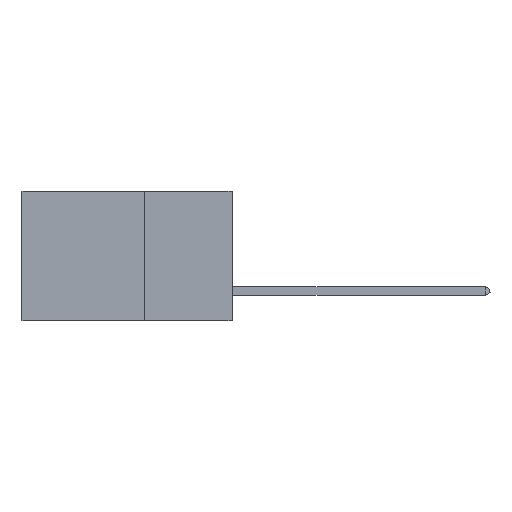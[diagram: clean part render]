
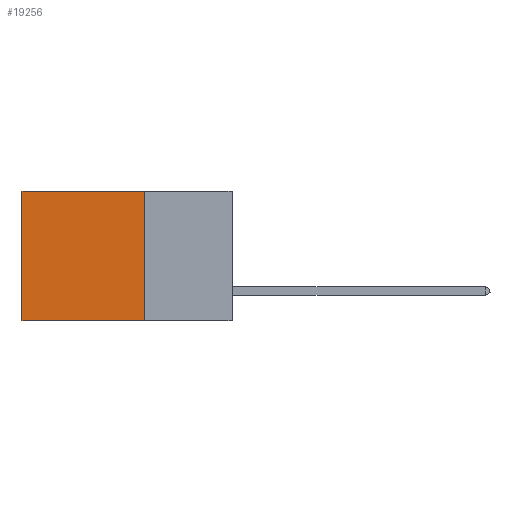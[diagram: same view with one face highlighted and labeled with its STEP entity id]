
A CAD part, left-side view. The second image highlights one B-rep face of the part: STEP entity #19256.
In plain terms, the highlighted planar face has unit normal (-1, 0, 0).
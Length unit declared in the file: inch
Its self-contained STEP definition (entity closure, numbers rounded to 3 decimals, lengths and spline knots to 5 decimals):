
#1192 = EDGE_LOOP ( 'NONE', ( #1279, #43005, #9288, #31970 ) ) ;
#1279 = ORIENTED_EDGE ( 'NONE', *, *, #7587, .T. ) ;
#2018 = CARTESIAN_POINT ( 'NONE',  ( 0.2875, 0.25, 0. ) ) ;
#5462 = AXIS2_PLACEMENT_3D ( 'NONE', #16844, #16388, #23739 ) ;
#7587 = EDGE_CURVE ( 'NONE', #22575, #18100, #30866, .T. ) ;
#8755 = DIRECTION ( 'NONE',  ( 0., 1., 0. ) ) ;
#9239 = DIRECTION ( 'NONE',  ( 0., 0., -1. ) ) ;
#9288 = ORIENTED_EDGE ( 'NONE', *, *, #26504, .F. ) ;
#16388 = DIRECTION ( 'NONE',  ( 1., 0., 0. ) ) ;
#16671 = LINE ( 'NONE', #2018, #36842 ) ;
#16844 = CARTESIAN_POINT ( 'NONE',  ( 0.2875, 0.25, 0. ) ) ;
#18100 = VERTEX_POINT ( 'NONE', #31803 ) ;
#18764 = VECTOR ( 'NONE', #8755, 39.37008 ) ;
#19256 = ADVANCED_FACE ( 'NONE', ( #23884 ), #38470, .F. ) ;
#19267 = DIRECTION ( 'NONE',  ( 0., 0., -1. ) ) ;
#22202 = DIRECTION ( 'NONE',  ( 0., 1., 0. ) ) ;
#22575 = VERTEX_POINT ( 'NONE', #42373 ) ;
#23262 = CARTESIAN_POINT ( 'NONE',  ( 0.2875, 0.25, -0.37 ) ) ;
#23739 = DIRECTION ( 'NONE',  ( 0., 0., -1. ) ) ;
#23884 = FACE_OUTER_BOUND ( 'NONE', #1192, .T. ) ;
#24040 = EDGE_CURVE ( 'NONE', #28176, #22575, #35311, .T. ) ;
#26504 = EDGE_CURVE ( 'NONE', #28176, #43264, #16671, .T. ) ;
#28176 = VERTEX_POINT ( 'NONE', #44977 ) ;
#29634 = CARTESIAN_POINT ( 'NONE',  ( 0.2875, 0.25, 0. ) ) ;
#30866 = LINE ( 'NONE', #41692, #43025 ) ;
#31803 = CARTESIAN_POINT ( 'NONE',  ( 0.2875, 0.6, -0.37 ) ) ;
#31970 = ORIENTED_EDGE ( 'NONE', *, *, #24040, .T. ) ;
#33189 = LINE ( 'NONE', #45816, #18764 ) ;
#35311 = LINE ( 'NONE', #29634, #37045 ) ;
#36842 = VECTOR ( 'NONE', #9239, 39.37008 ) ;
#37045 = VECTOR ( 'NONE', #22202, 39.37008 ) ;
#38470 = PLANE ( 'NONE',  #5462 ) ;
#41692 = CARTESIAN_POINT ( 'NONE',  ( 0.2875, 0.6, 0. ) ) ;
#42373 = CARTESIAN_POINT ( 'NONE',  ( 0.2875, 0.6, 0. ) ) ;
#43005 = ORIENTED_EDGE ( 'NONE', *, *, #47089, .F. ) ;
#43025 = VECTOR ( 'NONE', #19267, 39.37008 ) ;
#43264 = VERTEX_POINT ( 'NONE', #23262 ) ;
#44977 = CARTESIAN_POINT ( 'NONE',  ( 0.2875, 0.25, 0. ) ) ;
#45816 = CARTESIAN_POINT ( 'NONE',  ( 0.2875, 0.25, -0.37 ) ) ;
#47089 = EDGE_CURVE ( 'NONE', #43264, #18100, #33189, .T. ) ;
